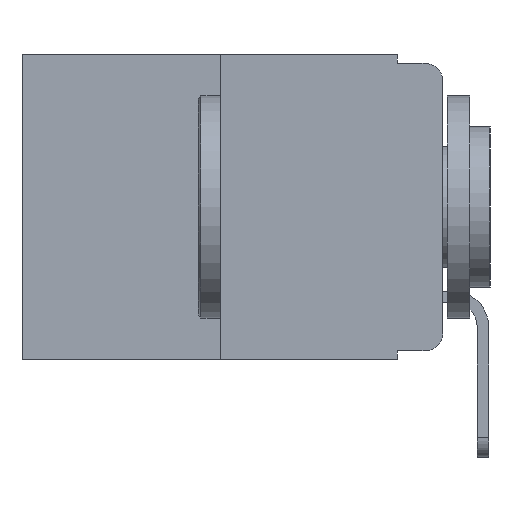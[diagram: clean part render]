
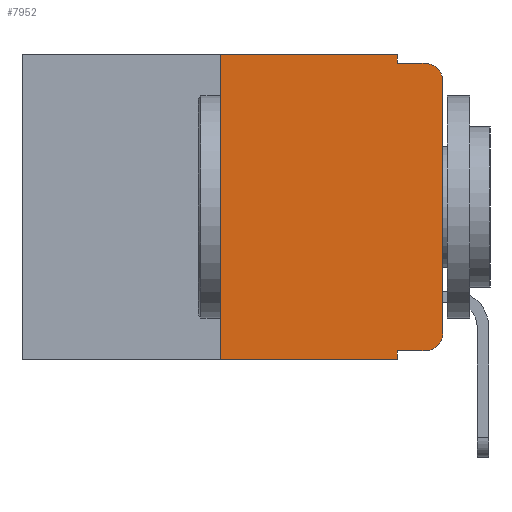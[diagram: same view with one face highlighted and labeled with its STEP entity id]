
A CAD part, left-side view. The second image highlights one B-rep face of the part: STEP entity #7952.
In plain terms, the highlighted planar face has unit normal (-1, 0, 0).
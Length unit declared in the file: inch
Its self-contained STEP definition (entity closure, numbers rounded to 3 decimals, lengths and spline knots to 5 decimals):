
#16 = EDGE_CURVE ( 'NONE', #14964, #15630, #20837, .T. ) ;
#225 = VECTOR ( 'NONE', #9706, 39.37008 ) ;
#427 = EDGE_CURVE ( 'NONE', #14387, #14964, #13911, .T. ) ;
#527 = ORIENTED_EDGE ( 'NONE', *, *, #16, .T. ) ;
#551 = VERTEX_POINT ( 'NONE', #4388 ) ;
#584 = EDGE_CURVE ( 'NONE', #18905, #14387, #5615, .T. ) ;
#1386 = DIRECTION ( 'NONE',  ( 0., 0., 1. ) ) ;
#1934 = VERTEX_POINT ( 'NONE', #2347 ) ;
#2012 = VERTEX_POINT ( 'NONE', #21829 ) ;
#2347 = CARTESIAN_POINT ( 'NONE',  ( 0., 0.051, -0.333 ) ) ;
#2685 = VECTOR ( 'NONE', #4422, 39.37008 ) ;
#2895 = DIRECTION ( 'NONE',  ( 1., 0., 0. ) ) ;
#3646 = ORIENTED_EDGE ( 'NONE', *, *, #4677, .F. ) ;
#3901 = LINE ( 'NONE', #10666, #17585 ) ;
#3979 = VERTEX_POINT ( 'NONE', #9131 ) ;
#4334 = CARTESIAN_POINT ( 'NONE',  ( 0., 0.473, -0.343 ) ) ;
#4388 = CARTESIAN_POINT ( 'NONE',  ( 0., 0.25, -0.343 ) ) ;
#4418 = CARTESIAN_POINT ( 'NONE',  ( 0., 0.02, -0.03 ) ) ;
#4422 = DIRECTION ( 'NONE',  ( 0., -1., 0. ) ) ;
#4677 = EDGE_CURVE ( 'NONE', #2012, #15630, #22211, .T. ) ;
#4886 = CARTESIAN_POINT ( 'NONE',  ( 0., 0.473, 0. ) ) ;
#5615 = CIRCLE ( 'NONE', #17751, 0.02 ) ;
#5963 = LINE ( 'NONE', #23416, #16991 ) ;
#6397 = VECTOR ( 'NONE', #15276, 39.37008 ) ;
#6895 = CARTESIAN_POINT ( 'NONE',  ( 0., 0.051, 0. ) ) ;
#6982 = CARTESIAN_POINT ( 'NONE',  ( 0., 0.051, -0.01 ) ) ;
#7452 = EDGE_LOOP ( 'NONE', ( #19821, #527, #3646, #17504, #7466, #10956, #9261, #7838, #8715, #21101 ) ) ;
#7466 = ORIENTED_EDGE ( 'NONE', *, *, #15753, .F. ) ;
#7587 = VECTOR ( 'NONE', #18507, 39.37008 ) ;
#7820 = LINE ( 'NONE', #18538, #16189 ) ;
#7838 = ORIENTED_EDGE ( 'NONE', *, *, #16381, .F. ) ;
#7952 = ADVANCED_FACE ( 'NONE', ( #19656 ), #14270, .F. ) ;
#8341 = CARTESIAN_POINT ( 'NONE',  ( 0., 0.02, -0.313 ) ) ;
#8715 = ORIENTED_EDGE ( 'NONE', *, *, #12699, .T. ) ;
#9033 = DIRECTION ( 'NONE',  ( 0., 0., -1. ) ) ;
#9131 = CARTESIAN_POINT ( 'NONE',  ( 0., 0.051, -0.343 ) ) ;
#9224 = EDGE_CURVE ( 'NONE', #551, #3979, #9539, .T. ) ;
#9261 = ORIENTED_EDGE ( 'NONE', *, *, #9224, .T. ) ;
#9539 = LINE ( 'NONE', #4334, #2685 ) ;
#9706 = DIRECTION ( 'NONE',  ( 0., 0., 1. ) ) ;
#9770 = EDGE_CURVE ( 'NONE', #23024, #2012, #5963, .T. ) ;
#10666 = CARTESIAN_POINT ( 'NONE',  ( 0., 0.473, 0. ) ) ;
#10956 = ORIENTED_EDGE ( 'NONE', *, *, #21230, .F. ) ;
#10999 = LINE ( 'NONE', #14527, #21753 ) ;
#11929 = DIRECTION ( 'NONE',  ( -1., 0., 0. ) ) ;
#12186 = DIRECTION ( 'NONE',  ( 0., 0., -1. ) ) ;
#12699 = EDGE_CURVE ( 'NONE', #1934, #18905, #17724, .T. ) ;
#13447 = CARTESIAN_POINT ( 'NONE',  ( 0., 0., 0. ) ) ;
#13849 = CARTESIAN_POINT ( 'NONE',  ( 0., 0., -0.03 ) ) ;
#13911 = LINE ( 'NONE', #13447, #225 ) ;
#14270 = PLANE ( 'NONE',  #19483 ) ;
#14387 = VERTEX_POINT ( 'NONE', #22324 ) ;
#14400 = DIRECTION ( 'NONE',  ( 0., -1., 0. ) ) ;
#14527 = CARTESIAN_POINT ( 'NONE',  ( 0., 0.051, 0. ) ) ;
#14964 = VERTEX_POINT ( 'NONE', #13849 ) ;
#15276 = DIRECTION ( 'NONE',  ( 0., -1., 0. ) ) ;
#15630 = VERTEX_POINT ( 'NONE', #19692 ) ;
#15753 = EDGE_CURVE ( 'NONE', #19055, #23024, #3901, .T. ) ;
#15973 = DIRECTION ( 'NONE',  ( 0., 0., -1. ) ) ;
#16189 = VECTOR ( 'NONE', #1386, 39.37008 ) ;
#16381 = EDGE_CURVE ( 'NONE', #1934, #3979, #10999, .T. ) ;
#16889 = CARTESIAN_POINT ( 'NONE',  ( 0., 0.25, 0. ) ) ;
#16991 = VECTOR ( 'NONE', #17734, 39.37008 ) ;
#17504 = ORIENTED_EDGE ( 'NONE', *, *, #9770, .F. ) ;
#17585 = VECTOR ( 'NONE', #14400, 39.37008 ) ;
#17724 = LINE ( 'NONE', #20649, #6397 ) ;
#17734 = DIRECTION ( 'NONE',  ( 0., 0., -1. ) ) ;
#17751 = AXIS2_PLACEMENT_3D ( 'NONE', #8341, #11929, #12186 ) ;
#18229 = DIRECTION ( 'NONE',  ( 0., 0., -1. ) ) ;
#18507 = DIRECTION ( 'NONE',  ( 0., -1., 0. ) ) ;
#18538 = CARTESIAN_POINT ( 'NONE',  ( 0., 0.25, 0. ) ) ;
#18905 = VERTEX_POINT ( 'NONE', #21667 ) ;
#19055 = VERTEX_POINT ( 'NONE', #16889 ) ;
#19483 = AXIS2_PLACEMENT_3D ( 'NONE', #4886, #2895, #18229 ) ;
#19656 = FACE_OUTER_BOUND ( 'NONE', #7452, .T. ) ;
#19662 = DIRECTION ( 'NONE',  ( -1., 0., 0. ) ) ;
#19692 = CARTESIAN_POINT ( 'NONE',  ( 0., 0.02, -0.01 ) ) ;
#19821 = ORIENTED_EDGE ( 'NONE', *, *, #427, .T. ) ;
#20649 = CARTESIAN_POINT ( 'NONE',  ( 0., 0.051, -0.333 ) ) ;
#20837 = CIRCLE ( 'NONE', #22092, 0.02 ) ;
#21101 = ORIENTED_EDGE ( 'NONE', *, *, #584, .T. ) ;
#21230 = EDGE_CURVE ( 'NONE', #551, #19055, #7820, .T. ) ;
#21667 = CARTESIAN_POINT ( 'NONE',  ( 0., 0.02, -0.333 ) ) ;
#21753 = VECTOR ( 'NONE', #9033, 39.37008 ) ;
#21829 = CARTESIAN_POINT ( 'NONE',  ( 0., 0.051, -0.01 ) ) ;
#22092 = AXIS2_PLACEMENT_3D ( 'NONE', #4418, #19662, #15973 ) ;
#22211 = LINE ( 'NONE', #6982, #7587 ) ;
#22324 = CARTESIAN_POINT ( 'NONE',  ( 0., 0., -0.313 ) ) ;
#23024 = VERTEX_POINT ( 'NONE', #6895 ) ;
#23416 = CARTESIAN_POINT ( 'NONE',  ( 0., 0.051, 0. ) ) ;
